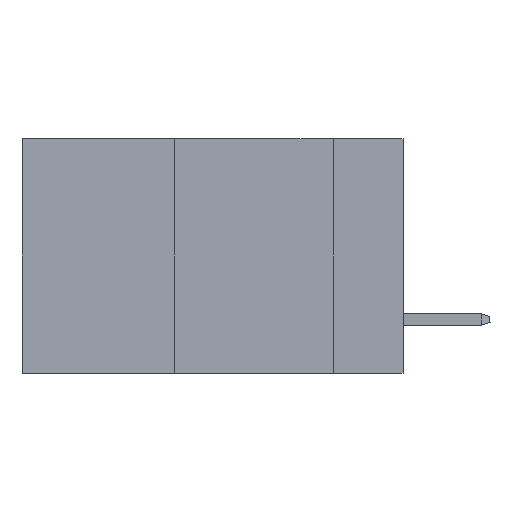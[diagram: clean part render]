
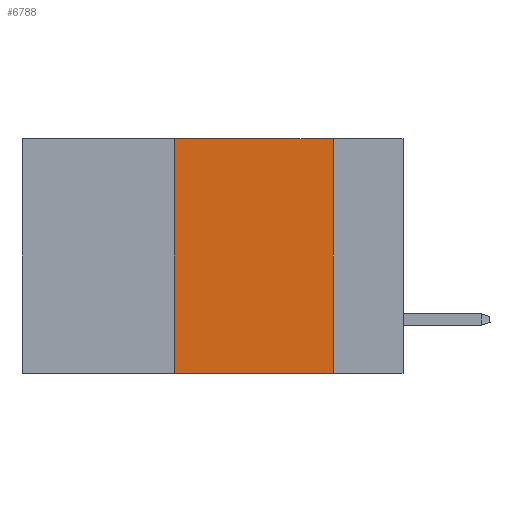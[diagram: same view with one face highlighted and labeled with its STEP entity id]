
A CAD part, left-side view. The second image highlights one B-rep face of the part: STEP entity #6788.
In plain terms, the highlighted planar face has unit normal (-1, 0, 0).
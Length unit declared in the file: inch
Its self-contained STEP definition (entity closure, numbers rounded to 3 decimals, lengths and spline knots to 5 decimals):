
#2285 = VECTOR ( 'NONE', #37578, 39.37008 ) ;
#4011 = EDGE_CURVE ( 'NONE', #22553, #4186, #18074, .T. ) ;
#4186 = VERTEX_POINT ( 'NONE', #9967 ) ;
#5341 = CARTESIAN_POINT ( 'NONE',  ( 0., 0.6, 0. ) ) ;
#6102 = VECTOR ( 'NONE', #22642, 39.37008 ) ;
#6788 = ADVANCED_FACE ( 'NONE', ( #32535 ), #11907, .F. ) ;
#8235 = ORIENTED_EDGE ( 'NONE', *, *, #16633, .T. ) ;
#9848 = VERTEX_POINT ( 'NONE', #13920 ) ;
#9967 = CARTESIAN_POINT ( 'NONE',  ( 0., 0.11, 0. ) ) ;
#11321 = DIRECTION ( 'NONE',  ( 0., 0., -1. ) ) ;
#11907 = PLANE ( 'NONE',  #28075 ) ;
#13920 = CARTESIAN_POINT ( 'NONE',  ( 0., 0.11, -0.37 ) ) ;
#14864 = ORIENTED_EDGE ( 'NONE', *, *, #24813, .F. ) ;
#15131 = DIRECTION ( 'NONE',  ( 0., -1., 0. ) ) ;
#16155 = CARTESIAN_POINT ( 'NONE',  ( 0., 0.6, -0.37 ) ) ;
#16633 = EDGE_CURVE ( 'NONE', #23869, #9848, #37003, .T. ) ;
#18074 = LINE ( 'NONE', #21446, #27806 ) ;
#20990 = DIRECTION ( 'NONE',  ( 1., 0., 0. ) ) ;
#21446 = CARTESIAN_POINT ( 'NONE',  ( 0., 0.6, 0. ) ) ;
#22079 = CARTESIAN_POINT ( 'NONE',  ( 0., 0.36, 0. ) ) ;
#22553 = VERTEX_POINT ( 'NONE', #26705 ) ;
#22642 = DIRECTION ( 'NONE',  ( 0., 0., -1. ) ) ;
#23869 = VERTEX_POINT ( 'NONE', #31325 ) ;
#24813 = EDGE_CURVE ( 'NONE', #23869, #22553, #29561, .T. ) ;
#26705 = CARTESIAN_POINT ( 'NONE',  ( 0., 0.36, 0. ) ) ;
#27336 = EDGE_LOOP ( 'NONE', ( #31402, #34192, #14864, #8235 ) ) ;
#27806 = VECTOR ( 'NONE', #15131, 39.37008 ) ;
#28075 = AXIS2_PLACEMENT_3D ( 'NONE', #5341, #20990, #11321 ) ;
#29371 = VECTOR ( 'NONE', #34617, 39.37008 ) ;
#29561 = LINE ( 'NONE', #22079, #2285 ) ;
#31325 = CARTESIAN_POINT ( 'NONE',  ( 0., 0.36, -0.37 ) ) ;
#31402 = ORIENTED_EDGE ( 'NONE', *, *, #38025, .F. ) ;
#31796 = CARTESIAN_POINT ( 'NONE',  ( 0., 0.11, 0. ) ) ;
#32535 = FACE_OUTER_BOUND ( 'NONE', #27336, .T. ) ;
#34192 = ORIENTED_EDGE ( 'NONE', *, *, #4011, .F. ) ;
#34195 = LINE ( 'NONE', #31796, #6102 ) ;
#34617 = DIRECTION ( 'NONE',  ( 0., -1., 0. ) ) ;
#37003 = LINE ( 'NONE', #16155, #29371 ) ;
#37578 = DIRECTION ( 'NONE',  ( 0., 0., 1. ) ) ;
#38025 = EDGE_CURVE ( 'NONE', #4186, #9848, #34195, .T. ) ;
